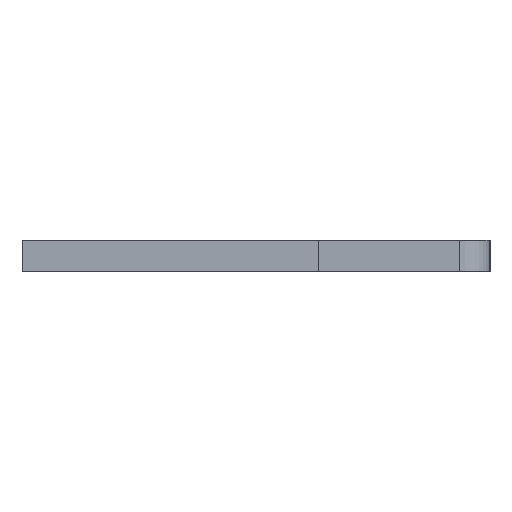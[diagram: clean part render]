
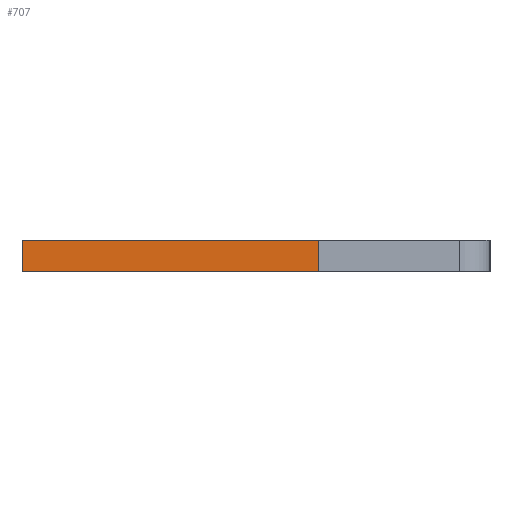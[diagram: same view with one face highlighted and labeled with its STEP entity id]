
A CAD part, left-side view. The second image highlights one B-rep face of the part: STEP entity #707.
In plain terms, the highlighted face is planar.
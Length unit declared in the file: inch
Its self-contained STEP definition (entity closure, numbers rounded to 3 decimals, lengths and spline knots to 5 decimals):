
#22 = VECTOR ( 'NONE', #413, 39.37008 ) ;
#51 = DIRECTION ( 'NONE',  ( 1., 0., 0. ) ) ;
#71 = CARTESIAN_POINT ( 'NONE',  ( 0.01, 0.15, -0.04 ) ) ;
#87 = EDGE_CURVE ( 'NONE', #430, #500, #840, .T. ) ;
#127 = CARTESIAN_POINT ( 'NONE',  ( -0.01, 0.15, -0.04 ) ) ;
#152 = VERTEX_POINT ( 'NONE', #965 ) ;
#250 = LINE ( 'NONE', #608, #772 ) ;
#411 = VECTOR ( 'NONE', #622, 39.37008 ) ;
#413 = DIRECTION ( 'NONE',  ( 0., 1., 0. ) ) ;
#428 = CARTESIAN_POINT ( 'NONE',  ( -0.01, -0.04, -0.04 ) ) ;
#430 = VERTEX_POINT ( 'NONE', #428 ) ;
#500 = VERTEX_POINT ( 'NONE', #127 ) ;
#525 = DIRECTION ( 'NONE',  ( 0., 0., 1. ) ) ;
#543 = FACE_OUTER_BOUND ( 'NONE', #842, .T. ) ;
#605 = DIRECTION ( 'NONE',  ( -1., 0., 0. ) ) ;
#606 = AXIS2_PLACEMENT_3D ( 'NONE', #912, #525, #51 ) ;
#608 = CARTESIAN_POINT ( 'NONE',  ( 0.01, 0.15, -0.04 ) ) ;
#622 = DIRECTION ( 'NONE',  ( -1., 0., 0. ) ) ;
#626 = CARTESIAN_POINT ( 'NONE',  ( 0.01, -0.04, -0.04 ) ) ;
#640 = ORIENTED_EDGE ( 'NONE', *, *, #675, .F. ) ;
#642 = CARTESIAN_POINT ( 'NONE',  ( -0.01, 0.15, -0.04 ) ) ;
#675 = EDGE_CURVE ( 'NONE', #887, #500, #250, .T. ) ;
#681 = PLANE ( 'NONE',  #606 ) ;
#707 = ADVANCED_FACE ( 'NONE', ( #543 ), #681, .F. ) ;
#772 = VECTOR ( 'NONE', #605, 39.37008 ) ;
#784 = EDGE_CURVE ( 'NONE', #152, #430, #858, .T. ) ;
#805 = LINE ( 'NONE', #1012, #897 ) ;
#833 = EDGE_CURVE ( 'NONE', #152, #887, #805, .T. ) ;
#840 = LINE ( 'NONE', #642, #22 ) ;
#842 = EDGE_LOOP ( 'NONE', ( #1022, #640, #1014, #877 ) ) ;
#858 = LINE ( 'NONE', #626, #411 ) ;
#877 = ORIENTED_EDGE ( 'NONE', *, *, #784, .T. ) ;
#887 = VERTEX_POINT ( 'NONE', #71 ) ;
#897 = VECTOR ( 'NONE', #1017, 39.37008 ) ;
#912 = CARTESIAN_POINT ( 'NONE',  ( 0.01, 0.15, -0.04 ) ) ;
#965 = CARTESIAN_POINT ( 'NONE',  ( 0.01, -0.04, -0.04 ) ) ;
#1012 = CARTESIAN_POINT ( 'NONE',  ( 0.01, 0.15, -0.04 ) ) ;
#1014 = ORIENTED_EDGE ( 'NONE', *, *, #833, .F. ) ;
#1017 = DIRECTION ( 'NONE',  ( 0., 1., 0. ) ) ;
#1022 = ORIENTED_EDGE ( 'NONE', *, *, #87, .T. ) ;
